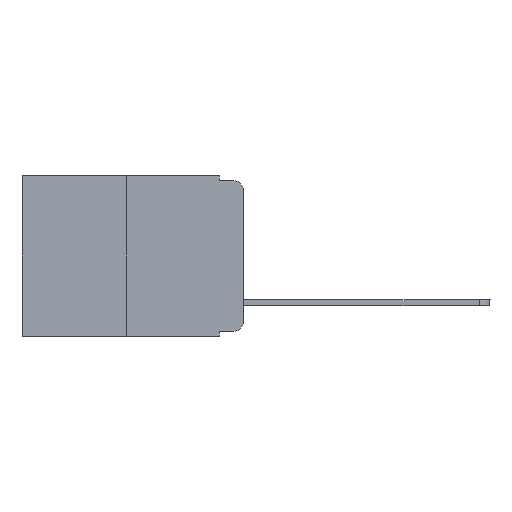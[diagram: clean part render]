
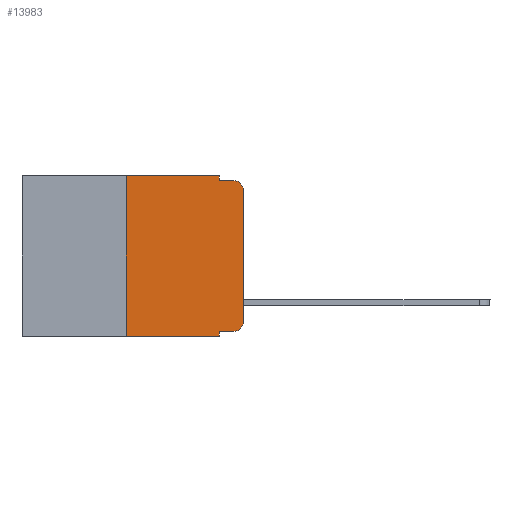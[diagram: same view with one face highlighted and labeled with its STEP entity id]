
A CAD part, left-side view. The second image highlights one B-rep face of the part: STEP entity #13983.
In plain terms, the highlighted planar face has unit normal (-1, 0, 0).
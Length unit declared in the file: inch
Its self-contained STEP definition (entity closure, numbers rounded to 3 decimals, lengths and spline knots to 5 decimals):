
#156 = VECTOR ( 'NONE', #5673, 39.37008 ) ;
#373 = LINE ( 'NONE', #665, #6330 ) ;
#418 = LINE ( 'NONE', #11571, #4419 ) ;
#590 = DIRECTION ( 'NONE',  ( 0., -1., 0. ) ) ;
#665 = CARTESIAN_POINT ( 'NONE',  ( 0., 0.473, -0.343 ) ) ;
#1235 = EDGE_LOOP ( 'NONE', ( #10187, #4723, #15236, #2081, #1479, #9954, #5736, #4258, #5088, #8939 ) ) ;
#1471 = VERTEX_POINT ( 'NONE', #6498 ) ;
#1479 = ORIENTED_EDGE ( 'NONE', *, *, #11115, .F. ) ;
#1731 = CARTESIAN_POINT ( 'NONE',  ( 0., 0.25, -0.343 ) ) ;
#1809 = VECTOR ( 'NONE', #11496, 39.37008 ) ;
#1896 = CIRCLE ( 'NONE', #3561, 0.02 ) ;
#2081 = ORIENTED_EDGE ( 'NONE', *, *, #14899, .F. ) ;
#2331 = CARTESIAN_POINT ( 'NONE',  ( 0., 0.051, -0.01 ) ) ;
#2456 = AXIS2_PLACEMENT_3D ( 'NONE', #4992, #7371, #8909 ) ;
#2835 = VERTEX_POINT ( 'NONE', #2904 ) ;
#2848 = DIRECTION ( 'NONE',  ( 0., 0., 1. ) ) ;
#2870 = VECTOR ( 'NONE', #5449, 39.37008 ) ;
#2904 = CARTESIAN_POINT ( 'NONE',  ( 0., 0.02, -0.333 ) ) ;
#3128 = CARTESIAN_POINT ( 'NONE',  ( 0., 0.051, 0. ) ) ;
#3157 = DIRECTION ( 'NONE',  ( 0., -1., 0. ) ) ;
#3561 = AXIS2_PLACEMENT_3D ( 'NONE', #15062, #10017, #3835 ) ;
#3835 = DIRECTION ( 'NONE',  ( 0., 0., -1. ) ) ;
#4004 = CARTESIAN_POINT ( 'NONE',  ( 0., 0.051, -0.343 ) ) ;
#4066 = CARTESIAN_POINT ( 'NONE',  ( 0., 0.051, -0.333 ) ) ;
#4249 = DIRECTION ( 'NONE',  ( 0., 0., -1. ) ) ;
#4258 = ORIENTED_EDGE ( 'NONE', *, *, #13001, .F. ) ;
#4359 = VERTEX_POINT ( 'NONE', #4004 ) ;
#4419 = VECTOR ( 'NONE', #15428, 39.37008 ) ;
#4723 = ORIENTED_EDGE ( 'NONE', *, *, #14104, .T. ) ;
#4992 = CARTESIAN_POINT ( 'NONE',  ( 0., 0.473, 0. ) ) ;
#5088 = ORIENTED_EDGE ( 'NONE', *, *, #8290, .T. ) ;
#5449 = DIRECTION ( 'NONE',  ( 0., 0., -1. ) ) ;
#5673 = DIRECTION ( 'NONE',  ( 0., 0., 1. ) ) ;
#5736 = ORIENTED_EDGE ( 'NONE', *, *, #7023, .T. ) ;
#5737 = VERTEX_POINT ( 'NONE', #14429 ) ;
#6330 = VECTOR ( 'NONE', #8188, 39.37008 ) ;
#6498 = CARTESIAN_POINT ( 'NONE',  ( 0., 0., -0.03 ) ) ;
#6601 = EDGE_CURVE ( 'NONE', #2835, #12871, #7894, .T. ) ;
#6893 = LINE ( 'NONE', #12890, #156 ) ;
#6897 = VERTEX_POINT ( 'NONE', #4066 ) ;
#7023 = EDGE_CURVE ( 'NONE', #11589, #4359, #373, .T. ) ;
#7371 = DIRECTION ( 'NONE',  ( 1., 0., 0. ) ) ;
#7395 = EDGE_CURVE ( 'NONE', #12871, #1471, #15284, .T. ) ;
#7894 = CIRCLE ( 'NONE', #13933, 0.02 ) ;
#8105 = CARTESIAN_POINT ( 'NONE',  ( 0., 0.02, -0.313 ) ) ;
#8188 = DIRECTION ( 'NONE',  ( 0., -1., 0. ) ) ;
#8246 = EDGE_CURVE ( 'NONE', #11589, #9123, #6893, .T. ) ;
#8290 = EDGE_CURVE ( 'NONE', #6897, #2835, #10487, .T. ) ;
#8456 = LINE ( 'NONE', #15202, #2870 ) ;
#8848 = VERTEX_POINT ( 'NONE', #3128 ) ;
#8909 = DIRECTION ( 'NONE',  ( 0., 0., -1. ) ) ;
#8939 = ORIENTED_EDGE ( 'NONE', *, *, #6601, .T. ) ;
#9015 = CARTESIAN_POINT ( 'NONE',  ( 0., 0., 0. ) ) ;
#9092 = CARTESIAN_POINT ( 'NONE',  ( 0., 0.051, -0.333 ) ) ;
#9123 = VERTEX_POINT ( 'NONE', #13673 ) ;
#9470 = VERTEX_POINT ( 'NONE', #2331 ) ;
#9647 = VECTOR ( 'NONE', #3157, 39.37008 ) ;
#9699 = EDGE_CURVE ( 'NONE', #9470, #5737, #12310, .T. ) ;
#9954 = ORIENTED_EDGE ( 'NONE', *, *, #8246, .F. ) ;
#10017 = DIRECTION ( 'NONE',  ( -1., 0., 0. ) ) ;
#10187 = ORIENTED_EDGE ( 'NONE', *, *, #7395, .T. ) ;
#10487 = LINE ( 'NONE', #9092, #10696 ) ;
#10488 = CARTESIAN_POINT ( 'NONE',  ( 0., 0.473, 0. ) ) ;
#10696 = VECTOR ( 'NONE', #590, 39.37008 ) ;
#11063 = VECTOR ( 'NONE', #2848, 39.37008 ) ;
#11115 = EDGE_CURVE ( 'NONE', #9123, #8848, #12660, .T. ) ;
#11496 = DIRECTION ( 'NONE',  ( 0., -1., 0. ) ) ;
#11536 = CARTESIAN_POINT ( 'NONE',  ( 0., 0.051, -0.01 ) ) ;
#11571 = CARTESIAN_POINT ( 'NONE',  ( 0., 0.051, 0. ) ) ;
#11589 = VERTEX_POINT ( 'NONE', #1731 ) ;
#12310 = LINE ( 'NONE', #11536, #1809 ) ;
#12660 = LINE ( 'NONE', #10488, #9647 ) ;
#12871 = VERTEX_POINT ( 'NONE', #14729 ) ;
#12890 = CARTESIAN_POINT ( 'NONE',  ( 0., 0.25, 0. ) ) ;
#13001 = EDGE_CURVE ( 'NONE', #6897, #4359, #418, .T. ) ;
#13673 = CARTESIAN_POINT ( 'NONE',  ( 0., 0.25, 0. ) ) ;
#13933 = AXIS2_PLACEMENT_3D ( 'NONE', #8105, #15214, #4249 ) ;
#13983 = ADVANCED_FACE ( 'NONE', ( #15496 ), #14589, .F. ) ;
#14104 = EDGE_CURVE ( 'NONE', #1471, #5737, #1896, .T. ) ;
#14429 = CARTESIAN_POINT ( 'NONE',  ( 0., 0.02, -0.01 ) ) ;
#14589 = PLANE ( 'NONE',  #2456 ) ;
#14729 = CARTESIAN_POINT ( 'NONE',  ( 0., 0., -0.313 ) ) ;
#14899 = EDGE_CURVE ( 'NONE', #8848, #9470, #8456, .T. ) ;
#15062 = CARTESIAN_POINT ( 'NONE',  ( 0., 0.02, -0.03 ) ) ;
#15202 = CARTESIAN_POINT ( 'NONE',  ( 0., 0.051, 0. ) ) ;
#15214 = DIRECTION ( 'NONE',  ( -1., 0., 0. ) ) ;
#15236 = ORIENTED_EDGE ( 'NONE', *, *, #9699, .F. ) ;
#15284 = LINE ( 'NONE', #9015, #11063 ) ;
#15428 = DIRECTION ( 'NONE',  ( 0., 0., -1. ) ) ;
#15496 = FACE_OUTER_BOUND ( 'NONE', #1235, .T. ) ;
